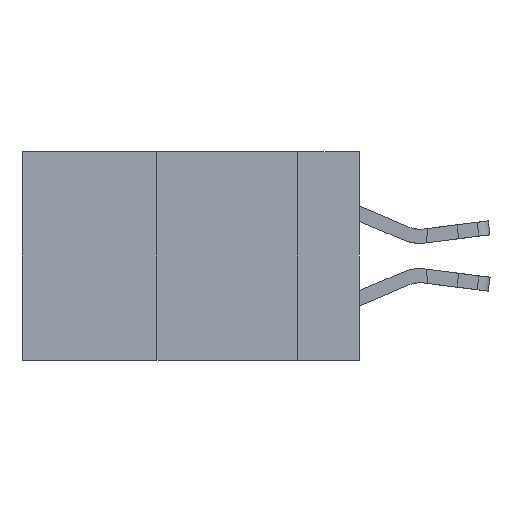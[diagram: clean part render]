
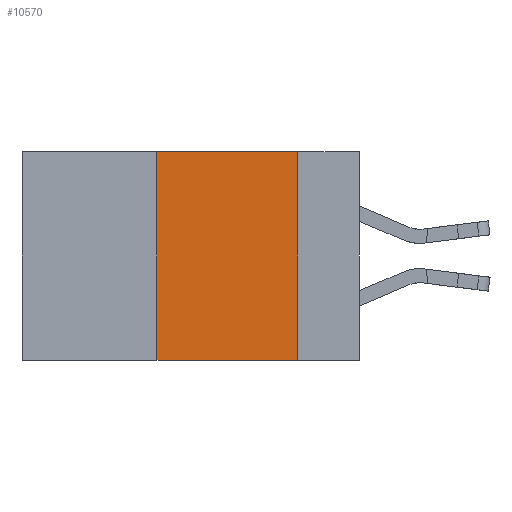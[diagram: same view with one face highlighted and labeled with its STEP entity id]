
A CAD part, left-side view. The second image highlights one B-rep face of the part: STEP entity #10570.
In plain terms, the highlighted planar face has unit normal (-1, 0, 0).
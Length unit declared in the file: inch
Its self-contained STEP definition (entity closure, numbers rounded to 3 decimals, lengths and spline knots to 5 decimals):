
#643 = EDGE_CURVE ( 'NONE', #20571, #21017, #20201, .T. ) ;
#1460 = CARTESIAN_POINT ( 'NONE',  ( 0., 0.36, 0. ) ) ;
#2481 = CARTESIAN_POINT ( 'NONE',  ( 0., 0.11, 0. ) ) ;
#2485 = PLANE ( 'NONE',  #12078 ) ;
#7742 = CARTESIAN_POINT ( 'NONE',  ( 0., 0.36, -0.37 ) ) ;
#8061 = LINE ( 'NONE', #8446, #16193 ) ;
#8439 = VECTOR ( 'NONE', #12460, 39.37008 ) ;
#8446 = CARTESIAN_POINT ( 'NONE',  ( 0., 0.6, 0. ) ) ;
#9389 = ORIENTED_EDGE ( 'NONE', *, *, #643, .F. ) ;
#10570 = ADVANCED_FACE ( 'NONE', ( #22949 ), #2485, .F. ) ;
#10933 = VERTEX_POINT ( 'NONE', #27082 ) ;
#12078 = AXIS2_PLACEMENT_3D ( 'NONE', #21483, #24386, #21774 ) ;
#12460 = DIRECTION ( 'NONE',  ( 0., -1., 0. ) ) ;
#13230 = LINE ( 'NONE', #19764, #8439 ) ;
#14162 = EDGE_CURVE ( 'NONE', #21017, #28357, #8061, .T. ) ;
#14509 = CARTESIAN_POINT ( 'NONE',  ( 0., 0.36, 0. ) ) ;
#16193 = VECTOR ( 'NONE', #27252, 39.37008 ) ;
#16977 = EDGE_LOOP ( 'NONE', ( #28640, #29530, #9389, #27204 ) ) ;
#18148 = EDGE_CURVE ( 'NONE', #20571, #10933, #13230, .T. ) ;
#18695 = VECTOR ( 'NONE', #19486, 39.37008 ) ;
#19434 = VECTOR ( 'NONE', #24184, 39.37008 ) ;
#19486 = DIRECTION ( 'NONE',  ( 0., 0., -1. ) ) ;
#19764 = CARTESIAN_POINT ( 'NONE',  ( 0., 0.6, -0.37 ) ) ;
#19831 = EDGE_CURVE ( 'NONE', #28357, #10933, #25020, .T. ) ;
#20201 = LINE ( 'NONE', #14509, #19434 ) ;
#20571 = VERTEX_POINT ( 'NONE', #7742 ) ;
#21017 = VERTEX_POINT ( 'NONE', #1460 ) ;
#21483 = CARTESIAN_POINT ( 'NONE',  ( 0., 0.6, 0. ) ) ;
#21774 = DIRECTION ( 'NONE',  ( 0., 0., -1. ) ) ;
#22949 = FACE_OUTER_BOUND ( 'NONE', #16977, .T. ) ;
#24184 = DIRECTION ( 'NONE',  ( 0., 0., 1. ) ) ;
#24386 = DIRECTION ( 'NONE',  ( 1., 0., 0. ) ) ;
#25020 = LINE ( 'NONE', #2481, #18695 ) ;
#27082 = CARTESIAN_POINT ( 'NONE',  ( 0., 0.11, -0.37 ) ) ;
#27204 = ORIENTED_EDGE ( 'NONE', *, *, #18148, .T. ) ;
#27252 = DIRECTION ( 'NONE',  ( 0., -1., 0. ) ) ;
#28357 = VERTEX_POINT ( 'NONE', #29111 ) ;
#28640 = ORIENTED_EDGE ( 'NONE', *, *, #19831, .F. ) ;
#29111 = CARTESIAN_POINT ( 'NONE',  ( 0., 0.11, 0. ) ) ;
#29530 = ORIENTED_EDGE ( 'NONE', *, *, #14162, .F. ) ;
